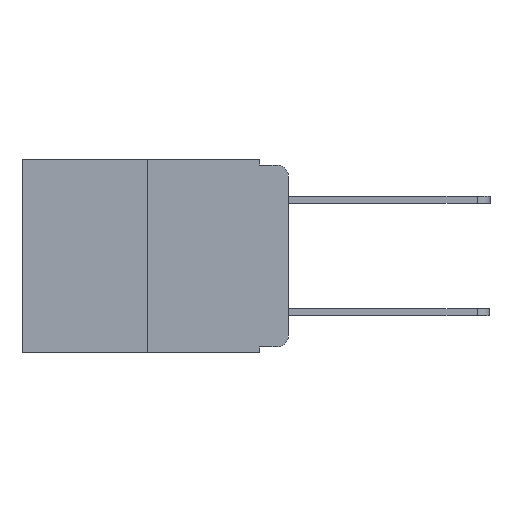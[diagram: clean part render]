
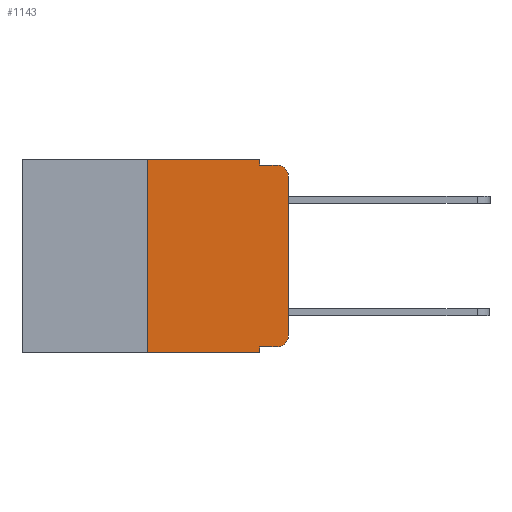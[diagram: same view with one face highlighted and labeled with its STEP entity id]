
A CAD part, left-side view. The second image highlights one B-rep face of the part: STEP entity #1143.
In plain terms, the highlighted planar face has unit normal (-1, 0, 0).
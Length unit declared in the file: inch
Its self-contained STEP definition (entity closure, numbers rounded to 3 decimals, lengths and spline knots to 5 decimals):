
#193 = LINE ( 'NONE', #13613, #5242 ) ;
#327 = VERTEX_POINT ( 'NONE', #10058 ) ;
#681 = CARTESIAN_POINT ( 'NONE',  ( 0., 0.25, 0. ) ) ;
#784 = VERTEX_POINT ( 'NONE', #13924 ) ;
#851 = CARTESIAN_POINT ( 'NONE',  ( 0., 0.051, 0. ) ) ;
#899 = LINE ( 'NONE', #851, #4873 ) ;
#1143 = ADVANCED_FACE ( 'NONE', ( #13077 ), #5622, .F. ) ;
#1260 = CARTESIAN_POINT ( 'NONE',  ( 0., 0., -0.03 ) ) ;
#1417 = AXIS2_PLACEMENT_3D ( 'NONE', #11601, #2815, #12881 ) ;
#1511 = EDGE_CURVE ( 'NONE', #2335, #10676, #193, .T. ) ;
#2335 = VERTEX_POINT ( 'NONE', #17542 ) ;
#2361 = VECTOR ( 'NONE', #9069, 39.37008 ) ;
#2585 = VERTEX_POINT ( 'NONE', #1260 ) ;
#2815 = DIRECTION ( 'NONE',  ( -1., 0., 0. ) ) ;
#2951 = CARTESIAN_POINT ( 'NONE',  ( 0., 0.02, -0.01 ) ) ;
#3057 = CARTESIAN_POINT ( 'NONE',  ( 0., 0.051, -0.01 ) ) ;
#3224 = VECTOR ( 'NONE', #14248, 39.37008 ) ;
#3397 = VERTEX_POINT ( 'NONE', #2951 ) ;
#3438 = VERTEX_POINT ( 'NONE', #7554 ) ;
#4100 = LINE ( 'NONE', #11648, #8980 ) ;
#4623 = CARTESIAN_POINT ( 'NONE',  ( 0., 0.051, 0. ) ) ;
#4873 = VECTOR ( 'NONE', #5794, 39.37008 ) ;
#5033 = EDGE_CURVE ( 'NONE', #13934, #3438, #8197, .T. ) ;
#5122 = AXIS2_PLACEMENT_3D ( 'NONE', #18066, #17600, #17396 ) ;
#5242 = VECTOR ( 'NONE', #16018, 39.37008 ) ;
#5322 = VERTEX_POINT ( 'NONE', #9547 ) ;
#5622 = PLANE ( 'NONE',  #5122 ) ;
#5794 = DIRECTION ( 'NONE',  ( 0., 0., -1. ) ) ;
#5954 = CIRCLE ( 'NONE', #6753, 0.02 ) ;
#6039 = CARTESIAN_POINT ( 'NONE',  ( 0., 0.051, -0.343 ) ) ;
#6048 = EDGE_CURVE ( 'NONE', #5322, #13934, #7465, .T. ) ;
#6373 = VECTOR ( 'NONE', #9071, 39.37008 ) ;
#6753 = AXIS2_PLACEMENT_3D ( 'NONE', #8932, #17716, #10339 ) ;
#6834 = CARTESIAN_POINT ( 'NONE',  ( 0., 0., 0. ) ) ;
#6997 = VECTOR ( 'NONE', #16212, 39.37008 ) ;
#7001 = EDGE_CURVE ( 'NONE', #5322, #10676, #899, .T. ) ;
#7465 = LINE ( 'NONE', #11178, #6997 ) ;
#7554 = CARTESIAN_POINT ( 'NONE',  ( 0., 0., -0.313 ) ) ;
#7976 = EDGE_CURVE ( 'NONE', #2335, #10446, #4100, .T. ) ;
#8197 = CIRCLE ( 'NONE', #1417, 0.02 ) ;
#8932 = CARTESIAN_POINT ( 'NONE',  ( 0., 0.02, -0.03 ) ) ;
#8980 = VECTOR ( 'NONE', #17721, 39.37008 ) ;
#9069 = DIRECTION ( 'NONE',  ( 0., -1., 0. ) ) ;
#9071 = DIRECTION ( 'NONE',  ( 0., 0., -1. ) ) ;
#9547 = CARTESIAN_POINT ( 'NONE',  ( 0., 0.051, -0.333 ) ) ;
#9922 = EDGE_CURVE ( 'NONE', #784, #327, #10630, .T. ) ;
#10040 = EDGE_LOOP ( 'NONE', ( #12843, #12839, #12672, #12627, #12559, #12281, #11986, #11969, #11829, #11826 ) ) ;
#10058 = CARTESIAN_POINT ( 'NONE',  ( 0., 0.051, -0.01 ) ) ;
#10196 = VECTOR ( 'NONE', #13649, 39.37008 ) ;
#10339 = DIRECTION ( 'NONE',  ( 0., 0., -1. ) ) ;
#10446 = VERTEX_POINT ( 'NONE', #681 ) ;
#10630 = LINE ( 'NONE', #4623, #6373 ) ;
#10676 = VERTEX_POINT ( 'NONE', #6039 ) ;
#10816 = LINE ( 'NONE', #15435, #2361 ) ;
#10823 = EDGE_CURVE ( 'NONE', #327, #3397, #11041, .T. ) ;
#11041 = LINE ( 'NONE', #3057, #3224 ) ;
#11178 = CARTESIAN_POINT ( 'NONE',  ( 0., 0.051, -0.333 ) ) ;
#11601 = CARTESIAN_POINT ( 'NONE',  ( 0., 0.02, -0.313 ) ) ;
#11648 = CARTESIAN_POINT ( 'NONE',  ( 0., 0.25, 0. ) ) ;
#11826 = ORIENTED_EDGE ( 'NONE', *, *, #5033, .T. ) ;
#11829 = ORIENTED_EDGE ( 'NONE', *, *, #6048, .T. ) ;
#11969 = ORIENTED_EDGE ( 'NONE', *, *, #7001, .F. ) ;
#11986 = ORIENTED_EDGE ( 'NONE', *, *, #1511, .T. ) ;
#12281 = ORIENTED_EDGE ( 'NONE', *, *, #7976, .F. ) ;
#12526 = EDGE_CURVE ( 'NONE', #2585, #3397, #5954, .T. ) ;
#12559 = ORIENTED_EDGE ( 'NONE', *, *, #14833, .F. ) ;
#12627 = ORIENTED_EDGE ( 'NONE', *, *, #9922, .F. ) ;
#12672 = ORIENTED_EDGE ( 'NONE', *, *, #10823, .F. ) ;
#12839 = ORIENTED_EDGE ( 'NONE', *, *, #12526, .T. ) ;
#12843 = ORIENTED_EDGE ( 'NONE', *, *, #14206, .T. ) ;
#12881 = DIRECTION ( 'NONE',  ( 0., 0., -1. ) ) ;
#13077 = FACE_OUTER_BOUND ( 'NONE', #10040, .T. ) ;
#13277 = CARTESIAN_POINT ( 'NONE',  ( 0., 0.02, -0.333 ) ) ;
#13598 = LINE ( 'NONE', #6834, #10196 ) ;
#13613 = CARTESIAN_POINT ( 'NONE',  ( 0., 0.473, -0.343 ) ) ;
#13649 = DIRECTION ( 'NONE',  ( 0., 0., 1. ) ) ;
#13924 = CARTESIAN_POINT ( 'NONE',  ( 0., 0.051, 0. ) ) ;
#13934 = VERTEX_POINT ( 'NONE', #13277 ) ;
#14206 = EDGE_CURVE ( 'NONE', #3438, #2585, #13598, .T. ) ;
#14248 = DIRECTION ( 'NONE',  ( 0., -1., 0. ) ) ;
#14833 = EDGE_CURVE ( 'NONE', #10446, #784, #10816, .T. ) ;
#15435 = CARTESIAN_POINT ( 'NONE',  ( 0., 0.473, 0. ) ) ;
#16018 = DIRECTION ( 'NONE',  ( 0., -1., 0. ) ) ;
#16212 = DIRECTION ( 'NONE',  ( 0., -1., 0. ) ) ;
#17396 = DIRECTION ( 'NONE',  ( 0., 0., -1. ) ) ;
#17542 = CARTESIAN_POINT ( 'NONE',  ( 0., 0.25, -0.343 ) ) ;
#17600 = DIRECTION ( 'NONE',  ( 1., 0., 0. ) ) ;
#17716 = DIRECTION ( 'NONE',  ( -1., 0., 0. ) ) ;
#17721 = DIRECTION ( 'NONE',  ( 0., 0., 1. ) ) ;
#18066 = CARTESIAN_POINT ( 'NONE',  ( 0., 0.473, 0. ) ) ;
